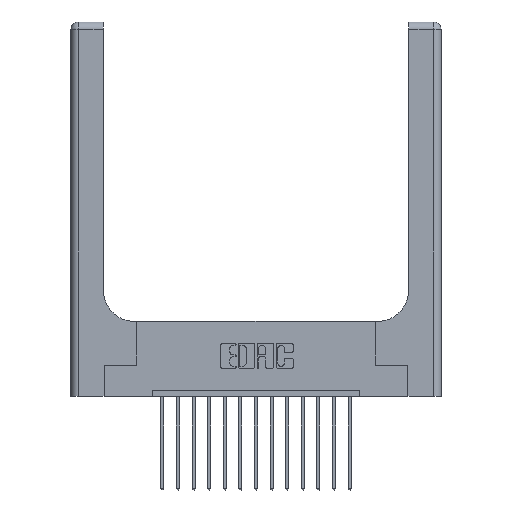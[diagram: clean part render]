
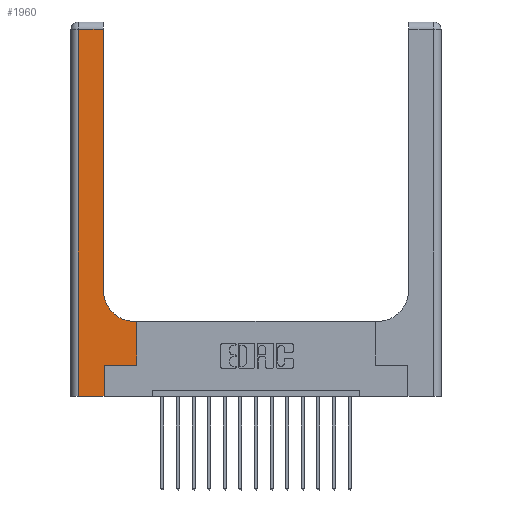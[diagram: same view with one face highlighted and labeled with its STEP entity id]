
A CAD part, top view. The second image highlights one B-rep face of the part: STEP entity #1960.
In plain terms, the highlighted planar face has unit normal (0, 0, 1).
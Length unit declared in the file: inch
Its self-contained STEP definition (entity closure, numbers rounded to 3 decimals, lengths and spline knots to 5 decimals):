
#30 = CARTESIAN_POINT ( 'NONE',  ( 0.528, 0.25, 0.37 ) ) ;
#342 = LINE ( 'NONE', #2592, #5319 ) ;
#480 = ORIENTED_EDGE ( 'NONE', *, *, #9950, .T. ) ;
#559 = CARTESIAN_POINT ( 'NONE',  ( 0.26, 0.85, 0.37 ) ) ;
#797 = DIRECTION ( 'NONE',  ( 0., 0., -1. ) ) ;
#977 = CARTESIAN_POINT ( 'NONE',  ( 0.26, 2.94, 0.37 ) ) ;
#1299 = EDGE_CURVE ( 'NONE', #7290, #5301, #15508, .T. ) ;
#1507 = VERTEX_POINT ( 'NONE', #8922 ) ;
#1932 = DIRECTION ( 'NONE',  ( 0., 1., 0. ) ) ;
#1960 = ADVANCED_FACE ( 'NONE', ( #13603 ), #13295, .F. ) ;
#2000 = CARTESIAN_POINT ( 'NONE',  ( 0., 2.94, 0.37 ) ) ;
#2010 = AXIS2_PLACEMENT_3D ( 'NONE', #3470, #797, #14312 ) ;
#2118 = EDGE_CURVE ( 'NONE', #8371, #4426, #12125, .T. ) ;
#2181 = DIRECTION ( 'NONE',  ( 1., 0., 0. ) ) ;
#2537 = VECTOR ( 'NONE', #14901, 39.37008 ) ;
#2592 = CARTESIAN_POINT ( 'NONE',  ( 0.06, 3., 0.37 ) ) ;
#2883 = CARTESIAN_POINT ( 'NONE',  ( 0.06, 2.94, 0.37 ) ) ;
#3470 = CARTESIAN_POINT ( 'NONE',  ( 0.51, 0.85, 0.37 ) ) ;
#3595 = EDGE_CURVE ( 'NONE', #1507, #7396, #12699, .T. ) ;
#3714 = ORIENTED_EDGE ( 'NONE', *, *, #3595, .T. ) ;
#3905 = VECTOR ( 'NONE', #1932, 39.37008 ) ;
#4113 = EDGE_CURVE ( 'NONE', #7396, #8371, #16425, .T. ) ;
#4117 = CARTESIAN_POINT ( 'NONE',  ( 0.265, 0.25, 0.37 ) ) ;
#4426 = VERTEX_POINT ( 'NONE', #30 ) ;
#4575 = EDGE_CURVE ( 'NONE', #4426, #14017, #14959, .T. ) ;
#4898 = VECTOR ( 'NONE', #14826, 39.37008 ) ;
#5301 = VERTEX_POINT ( 'NONE', #2883 ) ;
#5319 = VECTOR ( 'NONE', #10757, 39.37008 ) ;
#5592 = ORIENTED_EDGE ( 'NONE', *, *, #4113, .T. ) ;
#5792 = CARTESIAN_POINT ( 'NONE',  ( 0.265, 0., 0.37 ) ) ;
#5949 = CIRCLE ( 'NONE', #2010, 0.25 ) ;
#6341 = LINE ( 'NONE', #15064, #4898 ) ;
#6677 = VECTOR ( 'NONE', #15156, 39.37008 ) ;
#6837 = DIRECTION ( 'NONE',  ( 0., 1., 0. ) ) ;
#7290 = VERTEX_POINT ( 'NONE', #977 ) ;
#7396 = VERTEX_POINT ( 'NONE', #8618 ) ;
#7477 = CARTESIAN_POINT ( 'NONE',  ( 0.265, 0.25, 0.37 ) ) ;
#7692 = EDGE_LOOP ( 'NONE', ( #8566, #10121, #11254, #3714, #5592, #13276, #15345, #480, #12674 ) ) ;
#7867 = AXIS2_PLACEMENT_3D ( 'NONE', #14697, #14811, #8158 ) ;
#8158 = DIRECTION ( 'NONE',  ( -1., 0., 0. ) ) ;
#8257 = CARTESIAN_POINT ( 'NONE',  ( 0.528, 0.25, 0.37 ) ) ;
#8371 = VERTEX_POINT ( 'NONE', #7477 ) ;
#8566 = ORIENTED_EDGE ( 'NONE', *, *, #11816, .T. ) ;
#8618 = CARTESIAN_POINT ( 'NONE',  ( 0.265, 0., 0.37 ) ) ;
#8754 = VECTOR ( 'NONE', #2181, 39.37008 ) ;
#8922 = CARTESIAN_POINT ( 'NONE',  ( 0.06, 0., 0.37 ) ) ;
#9897 = EDGE_CURVE ( 'NONE', #5301, #1507, #342, .T. ) ;
#9950 = EDGE_CURVE ( 'NONE', #14017, #11827, #6341, .T. ) ;
#10121 = ORIENTED_EDGE ( 'NONE', *, *, #1299, .T. ) ;
#10455 = VECTOR ( 'NONE', #6837, 39.37008 ) ;
#10757 = DIRECTION ( 'NONE',  ( 0., -1., 0. ) ) ;
#11068 = CARTESIAN_POINT ( 'NONE',  ( 0.51, 0.6, 0.37 ) ) ;
#11254 = ORIENTED_EDGE ( 'NONE', *, *, #9897, .T. ) ;
#11707 = CARTESIAN_POINT ( 'NONE',  ( 0.528, 0.6, 0.37 ) ) ;
#11816 = EDGE_CURVE ( 'NONE', #15495, #7290, #11894, .T. ) ;
#11827 = VERTEX_POINT ( 'NONE', #11068 ) ;
#11835 = VECTOR ( 'NONE', #15051, 39.37008 ) ;
#11894 = LINE ( 'NONE', #15098, #10455 ) ;
#12125 = LINE ( 'NONE', #4117, #2537 ) ;
#12674 = ORIENTED_EDGE ( 'NONE', *, *, #14814, .T. ) ;
#12699 = LINE ( 'NONE', #16772, #8754 ) ;
#13276 = ORIENTED_EDGE ( 'NONE', *, *, #2118, .T. ) ;
#13295 = PLANE ( 'NONE',  #7867 ) ;
#13603 = FACE_OUTER_BOUND ( 'NONE', #7692, .T. ) ;
#14017 = VERTEX_POINT ( 'NONE', #11707 ) ;
#14312 = DIRECTION ( 'NONE',  ( 1., 0., 0. ) ) ;
#14697 = CARTESIAN_POINT ( 'NONE',  ( 0., 3., 0.37 ) ) ;
#14811 = DIRECTION ( 'NONE',  ( 0., 0., -1. ) ) ;
#14814 = EDGE_CURVE ( 'NONE', #11827, #15495, #5949, .T. ) ;
#14826 = DIRECTION ( 'NONE',  ( -1., 0., 0. ) ) ;
#14901 = DIRECTION ( 'NONE',  ( 1., 0., 0. ) ) ;
#14959 = LINE ( 'NONE', #8257, #3905 ) ;
#15051 = DIRECTION ( 'NONE',  ( 0., 1., 0. ) ) ;
#15064 = CARTESIAN_POINT ( 'NONE',  ( 0.26, 0.6, 0.37 ) ) ;
#15098 = CARTESIAN_POINT ( 'NONE',  ( 0.26, 3., 0.37 ) ) ;
#15156 = DIRECTION ( 'NONE',  ( -1., 0., 0. ) ) ;
#15345 = ORIENTED_EDGE ( 'NONE', *, *, #4575, .T. ) ;
#15495 = VERTEX_POINT ( 'NONE', #559 ) ;
#15508 = LINE ( 'NONE', #2000, #6677 ) ;
#16425 = LINE ( 'NONE', #5792, #11835 ) ;
#16772 = CARTESIAN_POINT ( 'NONE',  ( 0., 0., 0.37 ) ) ;
